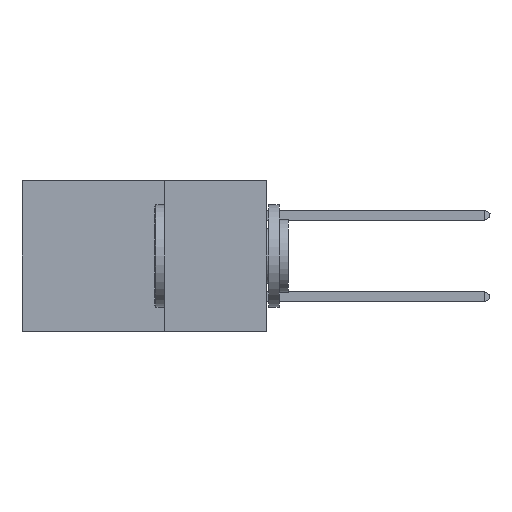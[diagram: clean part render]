
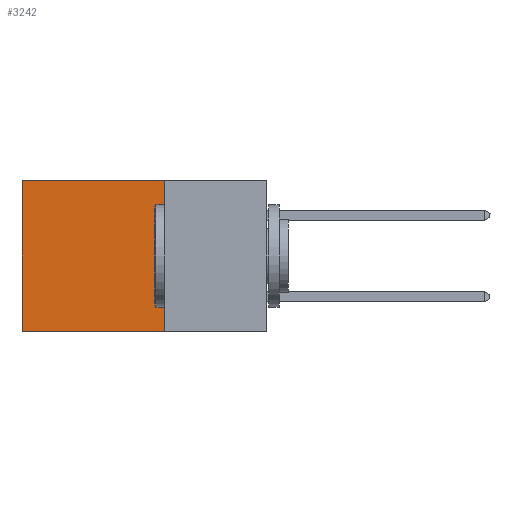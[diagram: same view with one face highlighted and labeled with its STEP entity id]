
A CAD part, left-side view. The second image highlights one B-rep face of the part: STEP entity #3242.
In plain terms, the highlighted planar face has unit normal (-1, 0, 0).
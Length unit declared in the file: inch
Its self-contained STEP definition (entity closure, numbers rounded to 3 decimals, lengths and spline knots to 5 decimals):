
#293 = CARTESIAN_POINT ( 'NONE',  ( 0.2875, 0.25, -0.37 ) ) ;
#2041 = CARTESIAN_POINT ( 'NONE',  ( 0.2875, 0.25, 0. ) ) ;
#3242 = ADVANCED_FACE ( 'NONE', ( #13919 ), #18353, .F. ) ;
#3969 = CARTESIAN_POINT ( 'NONE',  ( 0.2875, 0.25, 0. ) ) ;
#4314 = EDGE_CURVE ( 'NONE', #21704, #23473, #13195, .T. ) ;
#4329 = VERTEX_POINT ( 'NONE', #14468 ) ;
#5215 = LINE ( 'NONE', #22022, #14058 ) ;
#6421 = ORIENTED_EDGE ( 'NONE', *, *, #20878, .T. ) ;
#7687 = LINE ( 'NONE', #17007, #25094 ) ;
#11661 = EDGE_LOOP ( 'NONE', ( #28272, #18368, #16868, #6421 ) ) ;
#12423 = DIRECTION ( 'NONE',  ( 0., 1., 0. ) ) ;
#12577 = CARTESIAN_POINT ( 'NONE',  ( 0.2875, 0.6, -0.37 ) ) ;
#13195 = LINE ( 'NONE', #293, #18317 ) ;
#13391 = VERTEX_POINT ( 'NONE', #20422 ) ;
#13919 = FACE_OUTER_BOUND ( 'NONE', #11661, .T. ) ;
#14058 = VECTOR ( 'NONE', #29134, 39.37008 ) ;
#14468 = CARTESIAN_POINT ( 'NONE',  ( 0.2875, 0.6, 0. ) ) ;
#16868 = ORIENTED_EDGE ( 'NONE', *, *, #27767, .F. ) ;
#17007 = CARTESIAN_POINT ( 'NONE',  ( 0.2875, 0.25, 0. ) ) ;
#17450 = AXIS2_PLACEMENT_3D ( 'NONE', #3969, #17940, #27573 ) ;
#17940 = DIRECTION ( 'NONE',  ( 1., 0., 0. ) ) ;
#18317 = VECTOR ( 'NONE', #12423, 39.37008 ) ;
#18353 = PLANE ( 'NONE',  #17450 ) ;
#18368 = ORIENTED_EDGE ( 'NONE', *, *, #4314, .F. ) ;
#19134 = VECTOR ( 'NONE', #21328, 39.37008 ) ;
#20422 = CARTESIAN_POINT ( 'NONE',  ( 0.2875, 0.25, 0. ) ) ;
#20878 = EDGE_CURVE ( 'NONE', #13391, #4329, #7687, .T. ) ;
#21328 = DIRECTION ( 'NONE',  ( 0., 0., -1. ) ) ;
#21681 = CARTESIAN_POINT ( 'NONE',  ( 0.2875, 0.25, -0.37 ) ) ;
#21704 = VERTEX_POINT ( 'NONE', #21681 ) ;
#22022 = CARTESIAN_POINT ( 'NONE',  ( 0.2875, 0.6, 0. ) ) ;
#23473 = VERTEX_POINT ( 'NONE', #12577 ) ;
#24696 = LINE ( 'NONE', #2041, #19134 ) ;
#25094 = VECTOR ( 'NONE', #26063, 39.37008 ) ;
#25261 = EDGE_CURVE ( 'NONE', #4329, #23473, #5215, .T. ) ;
#26063 = DIRECTION ( 'NONE',  ( 0., 1., 0. ) ) ;
#27573 = DIRECTION ( 'NONE',  ( 0., 0., -1. ) ) ;
#27767 = EDGE_CURVE ( 'NONE', #13391, #21704, #24696, .T. ) ;
#28272 = ORIENTED_EDGE ( 'NONE', *, *, #25261, .T. ) ;
#29134 = DIRECTION ( 'NONE',  ( 0., 0., -1. ) ) ;
